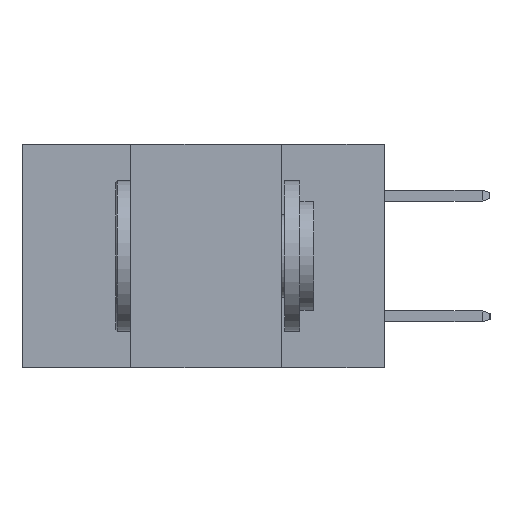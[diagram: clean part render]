
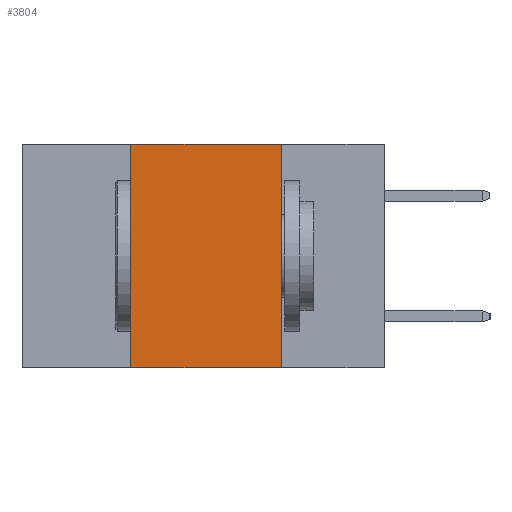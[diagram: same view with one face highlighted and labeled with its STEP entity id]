
A CAD part, left-side view. The second image highlights one B-rep face of the part: STEP entity #3804.
In plain terms, the highlighted planar face has unit normal (-1, 0, 0).
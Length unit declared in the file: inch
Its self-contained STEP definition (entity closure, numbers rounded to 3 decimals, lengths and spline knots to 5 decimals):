
#188 = VERTEX_POINT ( 'NONE', #10051 ) ;
#910 = PLANE ( 'NONE',  #3273 ) ;
#1312 = ORIENTED_EDGE ( 'NONE', *, *, #5159, .F. ) ;
#1512 = ORIENTED_EDGE ( 'NONE', *, *, #7620, .F. ) ;
#1874 = ORIENTED_EDGE ( 'NONE', *, *, #9967, .T. ) ;
#2244 = VERTEX_POINT ( 'NONE', #8963 ) ;
#2563 = LINE ( 'NONE', #12472, #8068 ) ;
#2801 = DIRECTION ( 'NONE',  ( 0., 0., -1. ) ) ;
#3273 = AXIS2_PLACEMENT_3D ( 'NONE', #13698, #13461, #2801 ) ;
#3760 = EDGE_LOOP ( 'NONE', ( #1512, #1312, #3847, #1874 ) ) ;
#3804 = ADVANCED_FACE ( 'NONE', ( #5363 ), #910, .F. ) ;
#3847 = ORIENTED_EDGE ( 'NONE', *, *, #8063, .F. ) ;
#5159 = EDGE_CURVE ( 'NONE', #13426, #188, #5170, .T. ) ;
#5170 = LINE ( 'NONE', #7649, #8392 ) ;
#5175 = VECTOR ( 'NONE', #8662, 39.37008 ) ;
#5363 = FACE_OUTER_BOUND ( 'NONE', #3760, .T. ) ;
#5467 = LINE ( 'NONE', #10878, #13655 ) ;
#6569 = CARTESIAN_POINT ( 'NONE',  ( 0., 0.42, -0.37 ) ) ;
#7477 = DIRECTION ( 'NONE',  ( 0., -1., 0. ) ) ;
#7620 = EDGE_CURVE ( 'NONE', #188, #2244, #2563, .T. ) ;
#7649 = CARTESIAN_POINT ( 'NONE',  ( 0., 0.6, 0. ) ) ;
#8056 = LINE ( 'NONE', #8937, #5175 ) ;
#8063 = EDGE_CURVE ( 'NONE', #8353, #13426, #8056, .T. ) ;
#8068 = VECTOR ( 'NONE', #12476, 39.37008 ) ;
#8353 = VERTEX_POINT ( 'NONE', #6569 ) ;
#8392 = VECTOR ( 'NONE', #7477, 39.37008 ) ;
#8662 = DIRECTION ( 'NONE',  ( 0., 0., 1. ) ) ;
#8937 = CARTESIAN_POINT ( 'NONE',  ( 0., 0.42, -0.37 ) ) ;
#8963 = CARTESIAN_POINT ( 'NONE',  ( 0., 0.17, -0.37 ) ) ;
#9967 = EDGE_CURVE ( 'NONE', #8353, #2244, #5467, .T. ) ;
#10051 = CARTESIAN_POINT ( 'NONE',  ( 0., 0.17, 0. ) ) ;
#10878 = CARTESIAN_POINT ( 'NONE',  ( 0., 0.6, -0.37 ) ) ;
#11928 = DIRECTION ( 'NONE',  ( 0., -1., 0. ) ) ;
#12472 = CARTESIAN_POINT ( 'NONE',  ( 0., 0.17, -0.37 ) ) ;
#12476 = DIRECTION ( 'NONE',  ( 0., 0., -1. ) ) ;
#13426 = VERTEX_POINT ( 'NONE', #13642 ) ;
#13461 = DIRECTION ( 'NONE',  ( 1., 0., 0. ) ) ;
#13642 = CARTESIAN_POINT ( 'NONE',  ( 0., 0.42, 0. ) ) ;
#13655 = VECTOR ( 'NONE', #11928, 39.37008 ) ;
#13698 = CARTESIAN_POINT ( 'NONE',  ( 0., 0.6, 0. ) ) ;
